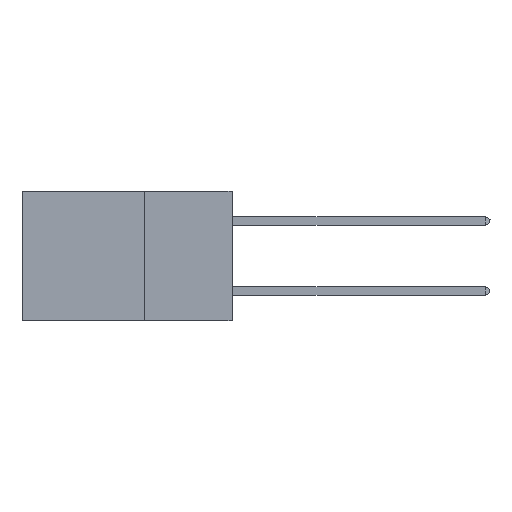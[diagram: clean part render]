
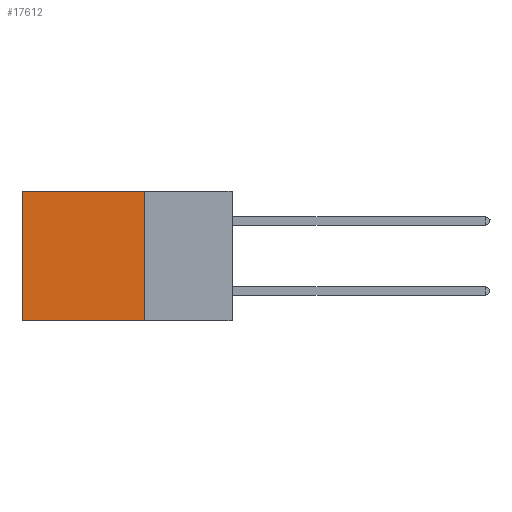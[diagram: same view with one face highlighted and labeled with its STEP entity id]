
A CAD part, left-side view. The second image highlights one B-rep face of the part: STEP entity #17612.
In plain terms, the highlighted planar face has unit normal (-1, 0, 0).
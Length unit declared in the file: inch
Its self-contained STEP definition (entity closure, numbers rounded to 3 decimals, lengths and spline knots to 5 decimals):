
#439 = CARTESIAN_POINT ( 'NONE',  ( 0.2875, 0.6, 0. ) ) ;
#3221 = DIRECTION ( 'NONE',  ( 0., 0., -1. ) ) ;
#4845 = CARTESIAN_POINT ( 'NONE',  ( 0.2875, 0.25, -0.37 ) ) ;
#5433 = CARTESIAN_POINT ( 'NONE',  ( 0.2875, 0.25, 0. ) ) ;
#6783 = PLANE ( 'NONE',  #26770 ) ;
#7220 = CARTESIAN_POINT ( 'NONE',  ( 0.2875, 0.25, 0. ) ) ;
#7466 = VECTOR ( 'NONE', #26017, 39.37008 ) ;
#8024 = ORIENTED_EDGE ( 'NONE', *, *, #21741, .F. ) ;
#8595 = LINE ( 'NONE', #439, #14149 ) ;
#9546 = DIRECTION ( 'NONE',  ( 0., 0., -1. ) ) ;
#9962 = VECTOR ( 'NONE', #26399, 39.37008 ) ;
#11238 = CARTESIAN_POINT ( 'NONE',  ( 0.2875, 0.6, 0. ) ) ;
#11369 = ORIENTED_EDGE ( 'NONE', *, *, #33439, .F. ) ;
#11611 = ORIENTED_EDGE ( 'NONE', *, *, #28428, .T. ) ;
#14149 = VECTOR ( 'NONE', #3221, 39.37008 ) ;
#16111 = EDGE_CURVE ( 'NONE', #17311, #18662, #8595, .T. ) ;
#16746 = ORIENTED_EDGE ( 'NONE', *, *, #16111, .T. ) ;
#17311 = VERTEX_POINT ( 'NONE', #11238 ) ;
#17612 = ADVANCED_FACE ( 'NONE', ( #23238 ), #6783, .F. ) ;
#18662 = VERTEX_POINT ( 'NONE', #30883 ) ;
#20351 = CARTESIAN_POINT ( 'NONE',  ( 0.2875, 0.25, 0. ) ) ;
#21741 = EDGE_CURVE ( 'NONE', #32067, #30005, #28038, .T. ) ;
#23238 = FACE_OUTER_BOUND ( 'NONE', #29980, .T. ) ;
#24323 = DIRECTION ( 'NONE',  ( 0., 1., 0. ) ) ;
#25381 = VECTOR ( 'NONE', #24323, 39.37008 ) ;
#25607 = DIRECTION ( 'NONE',  ( 1., 0., 0. ) ) ;
#26017 = DIRECTION ( 'NONE',  ( 0., 0., -1. ) ) ;
#26399 = DIRECTION ( 'NONE',  ( 0., 1., 0. ) ) ;
#26770 = AXIS2_PLACEMENT_3D ( 'NONE', #20351, #25607, #9546 ) ;
#28038 = LINE ( 'NONE', #7220, #7466 ) ;
#28428 = EDGE_CURVE ( 'NONE', #32067, #17311, #32382, .T. ) ;
#29980 = EDGE_LOOP ( 'NONE', ( #16746, #11369, #8024, #11611 ) ) ;
#30005 = VERTEX_POINT ( 'NONE', #33893 ) ;
#30883 = CARTESIAN_POINT ( 'NONE',  ( 0.2875, 0.6, -0.37 ) ) ;
#31244 = LINE ( 'NONE', #4845, #9962 ) ;
#32067 = VERTEX_POINT ( 'NONE', #33935 ) ;
#32382 = LINE ( 'NONE', #5433, #25381 ) ;
#33439 = EDGE_CURVE ( 'NONE', #30005, #18662, #31244, .T. ) ;
#33893 = CARTESIAN_POINT ( 'NONE',  ( 0.2875, 0.25, -0.37 ) ) ;
#33935 = CARTESIAN_POINT ( 'NONE',  ( 0.2875, 0.25, 0. ) ) ;
